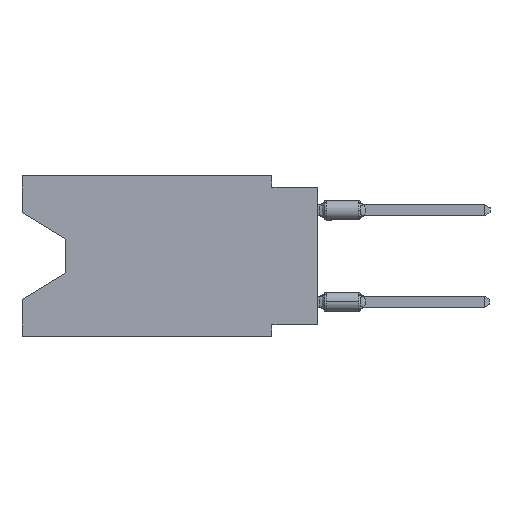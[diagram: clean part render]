
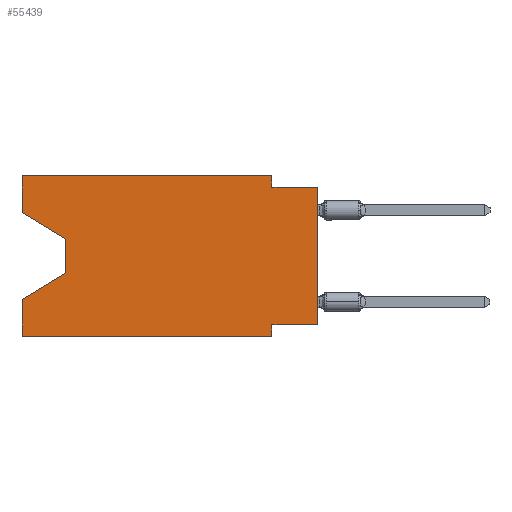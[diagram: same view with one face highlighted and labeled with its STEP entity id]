
A CAD part, left-side view. The second image highlights one B-rep face of the part: STEP entity #55439.
In plain terms, the highlighted planar face has unit normal (-1, 0, 0).
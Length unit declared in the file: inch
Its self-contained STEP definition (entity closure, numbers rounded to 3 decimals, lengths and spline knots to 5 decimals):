
#321 = ORIENTED_EDGE ( 'NONE', *, *, #50297, .F. ) ;
#583 = CARTESIAN_POINT ( 'NONE',  ( 0., 0.1, -0.025 ) ) ;
#619 = VECTOR ( 'NONE', #28062, 39.37008 ) ;
#3123 = DIRECTION ( 'NONE',  ( 0., -1., 0. ) ) ;
#4136 = EDGE_CURVE ( 'NONE', #46126, #6518, #50629, .T. ) ;
#4415 = PLANE ( 'NONE',  #6536 ) ;
#4702 = CARTESIAN_POINT ( 'NONE',  ( 0., 0.645, 0. ) ) ;
#5012 = DIRECTION ( 'NONE',  ( 0., 0., 1. ) ) ;
#5222 = EDGE_CURVE ( 'NONE', #42897, #33209, #54271, .T. ) ;
#5835 = CARTESIAN_POINT ( 'NONE',  ( 0., 0.645, 0. ) ) ;
#6518 = VERTEX_POINT ( 'NONE', #39650 ) ;
#6536 = AXIS2_PLACEMENT_3D ( 'NONE', #27278, #54640, #8345 ) ;
#7070 = DIRECTION ( 'NONE',  ( 0., 0., -1. ) ) ;
#7634 = LINE ( 'NONE', #12120, #43241 ) ;
#8345 = DIRECTION ( 'NONE',  ( 0., 0., -1. ) ) ;
#8476 = ORIENTED_EDGE ( 'NONE', *, *, #46676, .T. ) ;
#11977 = VECTOR ( 'NONE', #51421, 39.37008 ) ;
#12120 = CARTESIAN_POINT ( 'NONE',  ( 0., 0.645, -0.35 ) ) ;
#12747 = CARTESIAN_POINT ( 'NONE',  ( 0., 0.55, -0.138 ) ) ;
#13053 = CARTESIAN_POINT ( 'NONE',  ( 0., 0., -0.025 ) ) ;
#14135 = LINE ( 'NONE', #18962, #11977 ) ;
#16866 = VERTEX_POINT ( 'NONE', #47549 ) ;
#18385 = LINE ( 'NONE', #18683, #19733 ) ;
#18683 = CARTESIAN_POINT ( 'NONE',  ( 0., 0.55, -0.212 ) ) ;
#18804 = VECTOR ( 'NONE', #48209, 39.37008 ) ;
#18962 = CARTESIAN_POINT ( 'NONE',  ( 0., 0.645, 0. ) ) ;
#19068 = EDGE_CURVE ( 'NONE', #49416, #43639, #43881, .T. ) ;
#19515 = DIRECTION ( 'NONE',  ( 0., 0., -1. ) ) ;
#19733 = VECTOR ( 'NONE', #24044, 39.37008 ) ;
#19794 = CARTESIAN_POINT ( 'NONE',  ( 0., 0.1, 0. ) ) ;
#19862 = VERTEX_POINT ( 'NONE', #36695 ) ;
#20060 = CARTESIAN_POINT ( 'NONE',  ( 0., 0.645, -0.26975 ) ) ;
#20213 = VECTOR ( 'NONE', #5012, 39.37008 ) ;
#20495 = EDGE_CURVE ( 'NONE', #23242, #6518, #7634, .T. ) ;
#20908 = LINE ( 'NONE', #48291, #22292 ) ;
#21469 = VECTOR ( 'NONE', #19515, 39.37008 ) ;
#21866 = CARTESIAN_POINT ( 'NONE',  ( 0., 0.1, -0.325 ) ) ;
#21904 = DIRECTION ( 'NONE',  ( 0., -0.855, -0.519 ) ) ;
#22292 = VECTOR ( 'NONE', #7070, 39.37008 ) ;
#22896 = VERTEX_POINT ( 'NONE', #20060 ) ;
#23242 = VERTEX_POINT ( 'NONE', #37126 ) ;
#23586 = CARTESIAN_POINT ( 'NONE',  ( 0., 0.645, 0. ) ) ;
#23683 = EDGE_CURVE ( 'NONE', #23242, #22896, #47055, .T. ) ;
#24044 = DIRECTION ( 'NONE',  ( 0., 0.855, -0.519 ) ) ;
#24196 = DIRECTION ( 'NONE',  ( 0., 0., 1. ) ) ;
#24305 = LINE ( 'NONE', #19794, #21469 ) ;
#25124 = EDGE_CURVE ( 'NONE', #43639, #16866, #20908, .T. ) ;
#25677 = ORIENTED_EDGE ( 'NONE', *, *, #23683, .F. ) ;
#26986 = VECTOR ( 'NONE', #24196, 39.37008 ) ;
#27182 = EDGE_CURVE ( 'NONE', #56963, #42897, #24305, .T. ) ;
#27278 = CARTESIAN_POINT ( 'NONE',  ( 0., 0.645, 0. ) ) ;
#27934 = CARTESIAN_POINT ( 'NONE',  ( 0., 0., -0.025 ) ) ;
#28062 = DIRECTION ( 'NONE',  ( 0., 0., -1. ) ) ;
#29923 = ORIENTED_EDGE ( 'NONE', *, *, #27182, .F. ) ;
#30620 = EDGE_CURVE ( 'NONE', #34423, #56963, #14135, .T. ) ;
#31637 = ORIENTED_EDGE ( 'NONE', *, *, #30620, .F. ) ;
#32508 = ORIENTED_EDGE ( 'NONE', *, *, #25124, .T. ) ;
#33209 = VERTEX_POINT ( 'NONE', #27934 ) ;
#34423 = VERTEX_POINT ( 'NONE', #4702 ) ;
#35145 = CARTESIAN_POINT ( 'NONE',  ( 0., 0.645, -0.08025 ) ) ;
#35747 = FACE_OUTER_BOUND ( 'NONE', #46336, .T. ) ;
#36695 = CARTESIAN_POINT ( 'NONE',  ( 0., 0., -0.325 ) ) ;
#37087 = CARTESIAN_POINT ( 'NONE',  ( 0., 0.1, -0.35 ) ) ;
#37126 = CARTESIAN_POINT ( 'NONE',  ( 0., 0.645, -0.35 ) ) ;
#38365 = VECTOR ( 'NONE', #41071, 39.37008 ) ;
#39650 = CARTESIAN_POINT ( 'NONE',  ( 0., 0.1, -0.35 ) ) ;
#39868 = ORIENTED_EDGE ( 'NONE', *, *, #5222, .F. ) ;
#41071 = DIRECTION ( 'NONE',  ( 0., 0., 1. ) ) ;
#41910 = VECTOR ( 'NONE', #49773, 39.37008 ) ;
#42471 = ORIENTED_EDGE ( 'NONE', *, *, #4136, .F. ) ;
#42897 = VERTEX_POINT ( 'NONE', #583 ) ;
#43241 = VECTOR ( 'NONE', #3123, 39.37008 ) ;
#43639 = VERTEX_POINT ( 'NONE', #12747 ) ;
#43881 = LINE ( 'NONE', #35145, #53998 ) ;
#45916 = LINE ( 'NONE', #46214, #20213 ) ;
#46126 = VERTEX_POINT ( 'NONE', #21866 ) ;
#46214 = CARTESIAN_POINT ( 'NONE',  ( 0., 0., 0. ) ) ;
#46336 = EDGE_LOOP ( 'NONE', ( #51865, #32508, #8476, #25677, #57829, #42471, #51620, #49776, #39868, #29923, #31637, #321 ) ) ;
#46373 = EDGE_CURVE ( 'NONE', #19862, #46126, #52700, .T. ) ;
#46676 = EDGE_CURVE ( 'NONE', #16866, #22896, #18385, .T. ) ;
#47055 = LINE ( 'NONE', #5835, #26986 ) ;
#47296 = CARTESIAN_POINT ( 'NONE',  ( 0., 0., -0.325 ) ) ;
#47549 = CARTESIAN_POINT ( 'NONE',  ( 0., 0.55, -0.212 ) ) ;
#48209 = DIRECTION ( 'NONE',  ( 0., 1., 0. ) ) ;
#48291 = CARTESIAN_POINT ( 'NONE',  ( 0., 0.55, -0.138 ) ) ;
#49416 = VERTEX_POINT ( 'NONE', #51125 ) ;
#49773 = DIRECTION ( 'NONE',  ( 0., -1., 0. ) ) ;
#49776 = ORIENTED_EDGE ( 'NONE', *, *, #57515, .T. ) ;
#50297 = EDGE_CURVE ( 'NONE', #49416, #34423, #54591, .T. ) ;
#50629 = LINE ( 'NONE', #37087, #619 ) ;
#51125 = CARTESIAN_POINT ( 'NONE',  ( 0., 0.645, -0.08025 ) ) ;
#51421 = DIRECTION ( 'NONE',  ( 0., -1., 0. ) ) ;
#51620 = ORIENTED_EDGE ( 'NONE', *, *, #46373, .F. ) ;
#51865 = ORIENTED_EDGE ( 'NONE', *, *, #19068, .T. ) ;
#52700 = LINE ( 'NONE', #47296, #18804 ) ;
#53998 = VECTOR ( 'NONE', #21904, 39.37008 ) ;
#54271 = LINE ( 'NONE', #13053, #41910 ) ;
#54591 = LINE ( 'NONE', #23586, #38365 ) ;
#54640 = DIRECTION ( 'NONE',  ( 1., 0., 0. ) ) ;
#55439 = ADVANCED_FACE ( 'NONE', ( #35747 ), #4415, .F. ) ;
#55588 = CARTESIAN_POINT ( 'NONE',  ( 0., 0.1, 0. ) ) ;
#56963 = VERTEX_POINT ( 'NONE', #55588 ) ;
#57515 = EDGE_CURVE ( 'NONE', #19862, #33209, #45916, .T. ) ;
#57829 = ORIENTED_EDGE ( 'NONE', *, *, #20495, .T. ) ;
